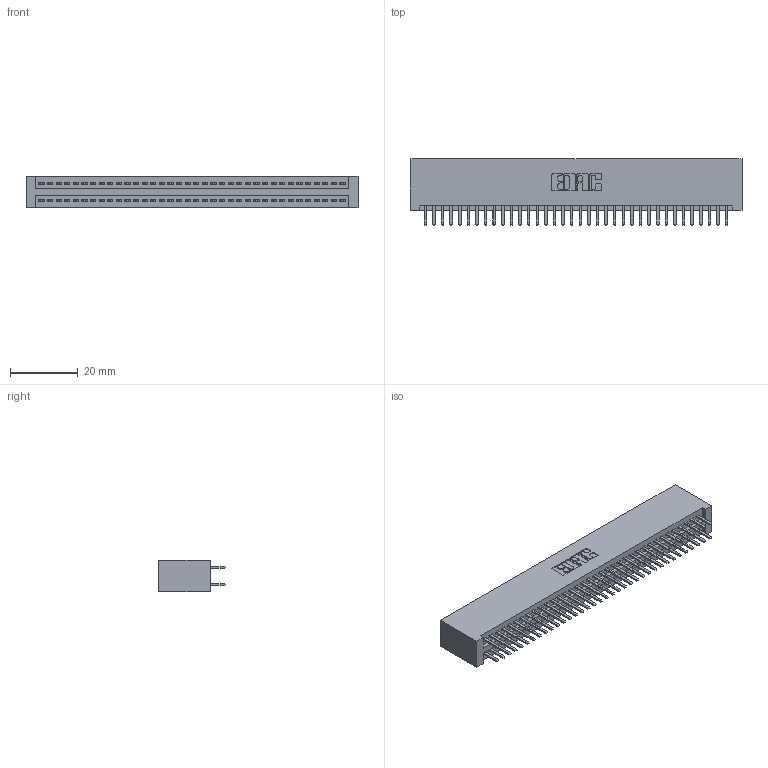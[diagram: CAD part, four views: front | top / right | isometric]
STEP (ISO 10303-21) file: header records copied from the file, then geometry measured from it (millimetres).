
FILE_DESCRIPTION (( 'STEP AP203' ), '1' );
FILE_NAME ('345-072-520-201.STEP', '2018-10-01T18:01:30', ( '' ), ( '' ), 'SwSTEP 2.0', 'SolidWorks 2016', '' );
FILE_SCHEMA (( 'CONFIG_CONTROL_DESIGN' ));
Length unit declared in the file: inch
Products named in the file (3): 345-072-520-201; 345-292-001_345-293-120; 345 Part_No Mounting Lugs
Assembly tree (73 placements, depth 2):
  345-072-520-201
    345 Part_No Mounting Lugs
    345-292-001_345-293-120  x72
Bounding box: 98.04 x 19.68 x 9.4 mm (x, y, z)
Volume: 10052.7 mm3; surface area: 14979.3 mm2
Topology: 73 solids, 73 shells, 4006 faces, 11621 edges, 7554 vertices
Faces by surface type: plane 2596, cylinder 1410
Entity records: 28891 total; most frequent: CARTESIAN_POINT 4860, ORIENTED_EDGE 4782, DIRECTION 4275, EDGE_CURVE 2391, VECTOR 2119, LINE 2119, VERTEX_POINT 1590, AXIS2_PLACEMENT_3D 1078
